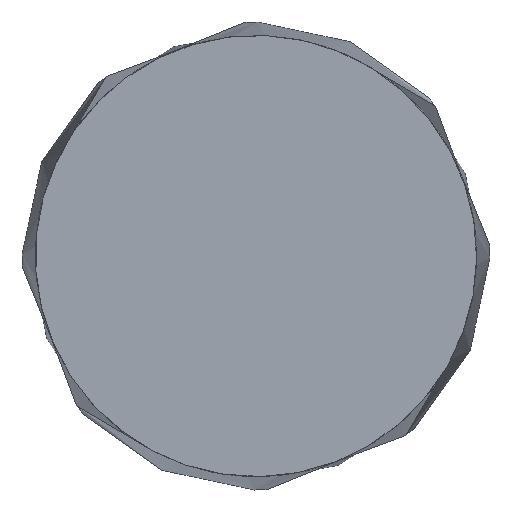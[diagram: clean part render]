
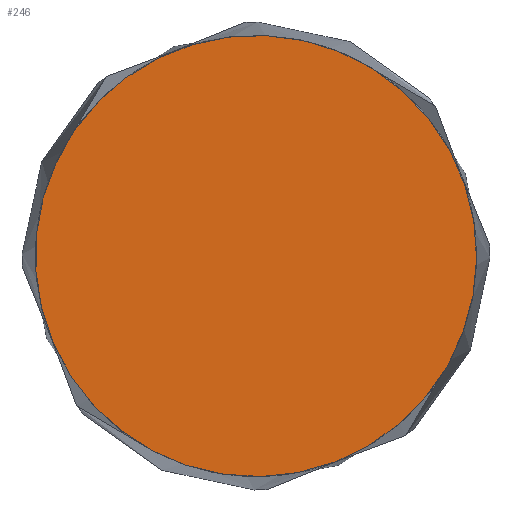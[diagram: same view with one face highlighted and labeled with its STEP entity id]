
A CAD part, left-side view. The second image highlights one B-rep face of the part: STEP entity #246.
In plain terms, the highlighted planar face has unit normal (-1, 0, 0).
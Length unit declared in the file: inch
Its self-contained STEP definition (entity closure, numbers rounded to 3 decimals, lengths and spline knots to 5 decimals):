
#45=PLANE('',#283);
#49=FACE_OUTER_BOUND('',#70,.T.);
#70=EDGE_LOOP('',(#175));
#89=CIRCLE('',#274,0.14764);
#109=VERTEX_POINT('',#358);
#129=EDGE_CURVE('',#109,#109,#89,.T.);
#175=ORIENTED_EDGE('',*,*,#129,.T.);
#246=ADVANCED_FACE('',(#49),#45,.F.);
#274=AXIS2_PLACEMENT_3D('',#359,#304,#305);
#283=AXIS2_PLACEMENT_3D('',#376,#322,#323);
#304=DIRECTION('center_axis',(-1.,0.,0.));
#305=DIRECTION('ref_axis',(0.,0.043,-0.999));
#322=DIRECTION('center_axis',(1.,0.,0.));
#323=DIRECTION('ref_axis',(0.,0.,-1.));
#358=CARTESIAN_POINT('',(-1.9685,-0.00639,0.1475));
#359=CARTESIAN_POINT('Origin',(-1.9685,0.,0.));
#376=CARTESIAN_POINT('Origin',(-1.9685,0.,0.));
